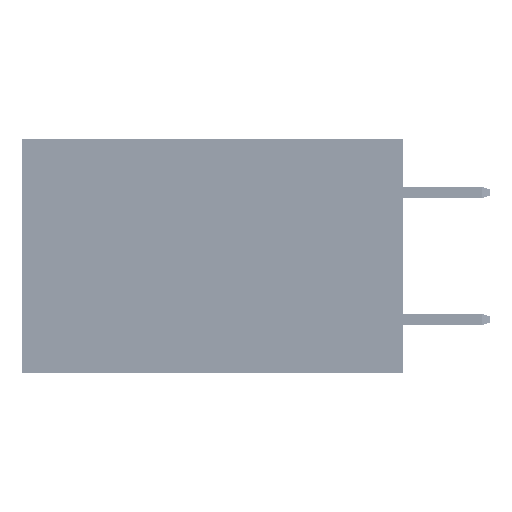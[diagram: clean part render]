
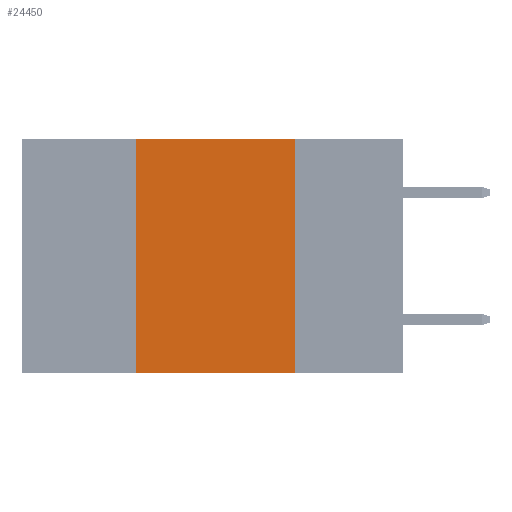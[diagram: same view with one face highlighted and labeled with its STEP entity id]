
A CAD part, left-side view. The second image highlights one B-rep face of the part: STEP entity #24450.
In plain terms, the highlighted planar face has unit normal (-1, 0, 0).
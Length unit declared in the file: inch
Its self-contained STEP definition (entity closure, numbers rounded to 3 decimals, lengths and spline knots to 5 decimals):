
#126 = ORIENTED_EDGE ( 'NONE', *, *, #44203, .F. ) ;
#2162 = VECTOR ( 'NONE', #40526, 39.37008 ) ;
#6042 = EDGE_LOOP ( 'NONE', ( #50958, #23208, #126, #38094 ) ) ;
#7843 = PLANE ( 'NONE',  #18421 ) ;
#7973 = VERTEX_POINT ( 'NONE', #40971 ) ;
#8565 = VECTOR ( 'NONE', #14539, 39.37008 ) ;
#9565 = CARTESIAN_POINT ( 'NONE',  ( 0., 0.42, 0. ) ) ;
#11284 = CARTESIAN_POINT ( 'NONE',  ( 0., 0.17, 0. ) ) ;
#12239 = FACE_OUTER_BOUND ( 'NONE', #6042, .T. ) ;
#12494 = CARTESIAN_POINT ( 'NONE',  ( 0., 0.6, 0. ) ) ;
#12923 = CARTESIAN_POINT ( 'NONE',  ( 0., 0.42, -0.37 ) ) ;
#14539 = DIRECTION ( 'NONE',  ( 0., -1., 0. ) ) ;
#15459 = CARTESIAN_POINT ( 'NONE',  ( 0., 0.17, 0. ) ) ;
#18421 = AXIS2_PLACEMENT_3D ( 'NONE', #12494, #23697, #32018 ) ;
#19365 = LINE ( 'NONE', #15459, #48098 ) ;
#20213 = CARTESIAN_POINT ( 'NONE',  ( 0., 0.6, 0. ) ) ;
#23208 = ORIENTED_EDGE ( 'NONE', *, *, #34809, .F. ) ;
#23295 = DIRECTION ( 'NONE',  ( 0., 0., -1. ) ) ;
#23571 = VERTEX_POINT ( 'NONE', #12923 ) ;
#23623 = VERTEX_POINT ( 'NONE', #9565 ) ;
#23697 = DIRECTION ( 'NONE',  ( 1., 0., 0. ) ) ;
#24165 = DIRECTION ( 'NONE',  ( 0., 0., 1. ) ) ;
#24450 = ADVANCED_FACE ( 'NONE', ( #12239 ), #7843, .F. ) ;
#26773 = VERTEX_POINT ( 'NONE', #11284 ) ;
#32018 = DIRECTION ( 'NONE',  ( 0., 0., -1. ) ) ;
#34809 = EDGE_CURVE ( 'NONE', #23623, #26773, #40020, .T. ) ;
#34866 = LINE ( 'NONE', #50761, #8565 ) ;
#38094 = ORIENTED_EDGE ( 'NONE', *, *, #49914, .T. ) ;
#39068 = EDGE_CURVE ( 'NONE', #26773, #7973, #19365, .T. ) ;
#40020 = LINE ( 'NONE', #20213, #2162 ) ;
#40312 = CARTESIAN_POINT ( 'NONE',  ( 0., 0.42, 0. ) ) ;
#40526 = DIRECTION ( 'NONE',  ( 0., -1., 0. ) ) ;
#40562 = LINE ( 'NONE', #40312, #50211 ) ;
#40971 = CARTESIAN_POINT ( 'NONE',  ( 0., 0.17, -0.37 ) ) ;
#44203 = EDGE_CURVE ( 'NONE', #23571, #23623, #40562, .T. ) ;
#48098 = VECTOR ( 'NONE', #23295, 39.37008 ) ;
#49914 = EDGE_CURVE ( 'NONE', #23571, #7973, #34866, .T. ) ;
#50211 = VECTOR ( 'NONE', #24165, 39.37008 ) ;
#50761 = CARTESIAN_POINT ( 'NONE',  ( 0., 0.6, -0.37 ) ) ;
#50958 = ORIENTED_EDGE ( 'NONE', *, *, #39068, .F. ) ;
